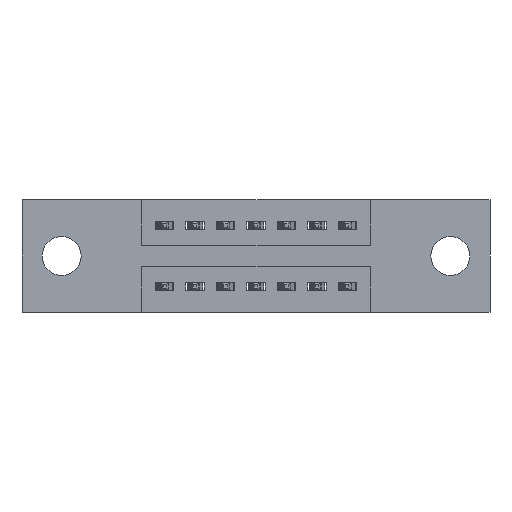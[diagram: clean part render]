
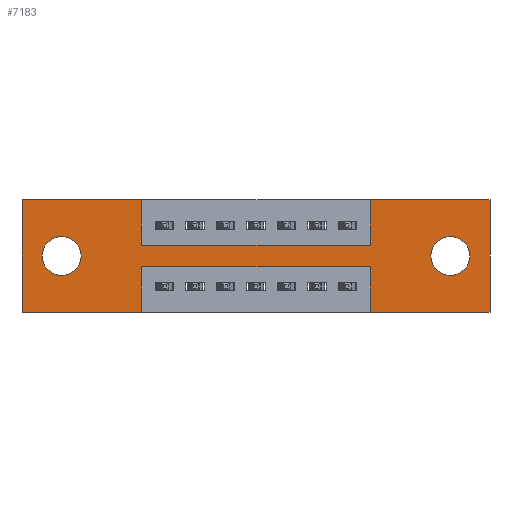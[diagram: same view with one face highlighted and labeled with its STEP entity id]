
A CAD part, front view. The second image highlights one B-rep face of the part: STEP entity #7183.
In plain terms, the highlighted planar face has unit normal (0, -1, 0).
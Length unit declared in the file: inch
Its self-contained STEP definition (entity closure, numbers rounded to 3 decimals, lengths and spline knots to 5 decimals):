
#76 = CARTESIAN_POINT ( 'NONE',  ( 1.535, 0., -0.37 ) ) ;
#187 = CARTESIAN_POINT ( 'NONE',  ( 1.405, 0., -0.121 ) ) ;
#204 = DIRECTION ( 'NONE',  ( 0., 0., 1. ) ) ;
#265 = AXIS2_PLACEMENT_3D ( 'NONE', #5460, #5365, #774 ) ;
#313 = ORIENTED_EDGE ( 'NONE', *, *, #1793, .T. ) ;
#326 = EDGE_CURVE ( 'NONE', #2442, #1435, #8876, .T. ) ;
#570 = EDGE_CURVE ( 'NONE', #6640, #3226, #3095, .T. ) ;
#571 = AXIS2_PLACEMENT_3D ( 'NONE', #7916, #8763, #7945 ) ;
#619 = ORIENTED_EDGE ( 'NONE', *, *, #6736, .F. ) ;
#620 = VECTOR ( 'NONE', #10150, 39.37008 ) ;
#634 = PLANE ( 'NONE',  #265 ) ;
#736 = VERTEX_POINT ( 'NONE', #3620 ) ;
#774 = DIRECTION ( 'NONE',  ( 0., 0., -1. ) ) ;
#858 = EDGE_CURVE ( 'NONE', #7406, #1645, #5656, .T. ) ;
#904 = ORIENTED_EDGE ( 'NONE', *, *, #1548, .F. ) ;
#1179 = EDGE_LOOP ( 'NONE', ( #6719, #5673 ) ) ;
#1204 = LINE ( 'NONE', #7947, #6472 ) ;
#1272 = VECTOR ( 'NONE', #204, 39.37008 ) ;
#1367 = CARTESIAN_POINT ( 'NONE',  ( 1.1425, 0., -0.22 ) ) ;
#1422 = VERTEX_POINT ( 'NONE', #1986 ) ;
#1435 = VERTEX_POINT ( 'NONE', #5290 ) ;
#1548 = EDGE_CURVE ( 'NONE', #7769, #8392, #8644, .T. ) ;
#1588 = VERTEX_POINT ( 'NONE', #10041 ) ;
#1621 = ORIENTED_EDGE ( 'NONE', *, *, #7367, .F. ) ;
#1645 = VERTEX_POINT ( 'NONE', #5626 ) ;
#1672 = EDGE_CURVE ( 'NONE', #1645, #3684, #1204, .T. ) ;
#1702 = DIRECTION ( 'NONE',  ( 0., 0., 1. ) ) ;
#1793 = EDGE_CURVE ( 'NONE', #3226, #6640, #6588, .T. ) ;
#1831 = VERTEX_POINT ( 'NONE', #4804 ) ;
#1974 = AXIS2_PLACEMENT_3D ( 'NONE', #4009, #9537, #6337 ) ;
#1986 = CARTESIAN_POINT ( 'NONE',  ( 1.1425, 0., 0. ) ) ;
#2091 = DIRECTION ( 'NONE',  ( -1., 0., 0. ) ) ;
#2158 = EDGE_CURVE ( 'NONE', #3633, #1831, #3235, .T. ) ;
#2379 = CARTESIAN_POINT ( 'NONE',  ( 0.3925, 0., -0.37 ) ) ;
#2424 = LINE ( 'NONE', #7381, #3416 ) ;
#2442 = VERTEX_POINT ( 'NONE', #76 ) ;
#2478 = DIRECTION ( 'NONE',  ( 0., 0., -1. ) ) ;
#2498 = AXIS2_PLACEMENT_3D ( 'NONE', #7168, #6262, #1702 ) ;
#2695 = LINE ( 'NONE', #8568, #620 ) ;
#2801 = AXIS2_PLACEMENT_3D ( 'NONE', #8997, #4231, #3451 ) ;
#3095 = CIRCLE ( 'NONE', #571, 0.064 ) ;
#3226 = VERTEX_POINT ( 'NONE', #5958 ) ;
#3235 = LINE ( 'NONE', #5209, #8972 ) ;
#3416 = VECTOR ( 'NONE', #6493, 39.37008 ) ;
#3451 = DIRECTION ( 'NONE',  ( 0., 0., 1. ) ) ;
#3563 = ORIENTED_EDGE ( 'NONE', *, *, #326, .F. ) ;
#3620 = CARTESIAN_POINT ( 'NONE',  ( 0.13, 0., -0.249 ) ) ;
#3630 = LINE ( 'NONE', #4315, #6886 ) ;
#3633 = VERTEX_POINT ( 'NONE', #4098 ) ;
#3645 = CARTESIAN_POINT ( 'NONE',  ( 0., 0., -0.37 ) ) ;
#3652 = VECTOR ( 'NONE', #7889, 39.37008 ) ;
#3684 = VERTEX_POINT ( 'NONE', #7980 ) ;
#3808 = ORIENTED_EDGE ( 'NONE', *, *, #9370, .F. ) ;
#3893 = DIRECTION ( 'NONE',  ( -1., 0., 0. ) ) ;
#4009 = CARTESIAN_POINT ( 'NONE',  ( 1.405, 0., -0.185 ) ) ;
#4098 = CARTESIAN_POINT ( 'NONE',  ( 0.3925, 0., -0.15 ) ) ;
#4099 = CARTESIAN_POINT ( 'NONE',  ( 0.13, 0., -0.121 ) ) ;
#4231 = DIRECTION ( 'NONE',  ( 0., 1., 0. ) ) ;
#4315 = CARTESIAN_POINT ( 'NONE',  ( 1.535, 0., 0. ) ) ;
#4366 = CARTESIAN_POINT ( 'NONE',  ( 0., 0., 0. ) ) ;
#4501 = CARTESIAN_POINT ( 'NONE',  ( 0.3925, 0., -0.22 ) ) ;
#4554 = FACE_BOUND ( 'NONE', #6823, .T. ) ;
#4710 = VECTOR ( 'NONE', #8277, 39.37008 ) ;
#4774 = DIRECTION ( 'NONE',  ( 0., 0., 1. ) ) ;
#4804 = CARTESIAN_POINT ( 'NONE',  ( 1.1425, 0., -0.15 ) ) ;
#5135 = VECTOR ( 'NONE', #2478, 39.37008 ) ;
#5209 = CARTESIAN_POINT ( 'NONE',  ( 0.3925, 0., -0.15 ) ) ;
#5290 = CARTESIAN_POINT ( 'NONE',  ( 1.1425, 0., -0.37 ) ) ;
#5318 = CARTESIAN_POINT ( 'NONE',  ( 0.3925, 0., -0.22 ) ) ;
#5365 = DIRECTION ( 'NONE',  ( 0., -1., 0. ) ) ;
#5398 = FACE_BOUND ( 'NONE', #1179, .T. ) ;
#5460 = CARTESIAN_POINT ( 'NONE',  ( 0., 0., -0.37 ) ) ;
#5626 = CARTESIAN_POINT ( 'NONE',  ( 0., 0., -0.37 ) ) ;
#5648 = CARTESIAN_POINT ( 'NONE',  ( 1.1425, 0., -0.37 ) ) ;
#5656 = LINE ( 'NONE', #5968, #7804 ) ;
#5673 = ORIENTED_EDGE ( 'NONE', *, *, #10101, .T. ) ;
#5956 = EDGE_CURVE ( 'NONE', #3684, #1588, #2424, .T. ) ;
#5958 = CARTESIAN_POINT ( 'NONE',  ( 1.405, 0., -0.249 ) ) ;
#5968 = CARTESIAN_POINT ( 'NONE',  ( 0., 0., -0.37 ) ) ;
#5972 = EDGE_CURVE ( 'NONE', #9496, #736, #7125, .T. ) ;
#6105 = ORIENTED_EDGE ( 'NONE', *, *, #570, .T. ) ;
#6245 = CIRCLE ( 'NONE', #2498, 0.064 ) ;
#6262 = DIRECTION ( 'NONE',  ( 0., 1., 0. ) ) ;
#6337 = DIRECTION ( 'NONE',  ( 0., 0., -1. ) ) ;
#6466 = VECTOR ( 'NONE', #10005, 39.37008 ) ;
#6472 = VECTOR ( 'NONE', #4774, 39.37008 ) ;
#6493 = DIRECTION ( 'NONE',  ( 1., 0., 0. ) ) ;
#6557 = LINE ( 'NONE', #5648, #1272 ) ;
#6588 = CIRCLE ( 'NONE', #1974, 0.064 ) ;
#6640 = VERTEX_POINT ( 'NONE', #187 ) ;
#6697 = DIRECTION ( 'NONE',  ( 0., 0., -1. ) ) ;
#6719 = ORIENTED_EDGE ( 'NONE', *, *, #5972, .T. ) ;
#6736 = EDGE_CURVE ( 'NONE', #1435, #7769, #6557, .T. ) ;
#6823 = EDGE_LOOP ( 'NONE', ( #6105, #313 ) ) ;
#6841 = ORIENTED_EDGE ( 'NONE', *, *, #5956, .F. ) ;
#6886 = VECTOR ( 'NONE', #6697, 39.37008 ) ;
#7125 = CIRCLE ( 'NONE', #2801, 0.064 ) ;
#7129 = ORIENTED_EDGE ( 'NONE', *, *, #858, .F. ) ;
#7168 = CARTESIAN_POINT ( 'NONE',  ( 0.13, 0., -0.185 ) ) ;
#7183 = ADVANCED_FACE ( 'NONE', ( #4554, #5398, #8300 ), #634, .T. ) ;
#7187 = ORIENTED_EDGE ( 'NONE', *, *, #1672, .F. ) ;
#7300 = CARTESIAN_POINT ( 'NONE',  ( 0.3925, 0., -0.37 ) ) ;
#7367 = EDGE_CURVE ( 'NONE', #1588, #3633, #8810, .T. ) ;
#7381 = CARTESIAN_POINT ( 'NONE',  ( 0., 0., 0. ) ) ;
#7406 = VERTEX_POINT ( 'NONE', #7300 ) ;
#7512 = EDGE_CURVE ( 'NONE', #1422, #9919, #10200, .T. ) ;
#7709 = EDGE_LOOP ( 'NONE', ( #8619, #904, #619, #3563, #3808, #7728, #8996, #8426, #1621, #6841, #7187, #7129 ) ) ;
#7728 = ORIENTED_EDGE ( 'NONE', *, *, #7512, .F. ) ;
#7769 = VERTEX_POINT ( 'NONE', #1367 ) ;
#7804 = VECTOR ( 'NONE', #2091, 39.37008 ) ;
#7873 = VECTOR ( 'NONE', #3893, 39.37008 ) ;
#7889 = DIRECTION ( 'NONE',  ( 0., 0., -1. ) ) ;
#7916 = CARTESIAN_POINT ( 'NONE',  ( 1.405, 0., -0.185 ) ) ;
#7945 = DIRECTION ( 'NONE',  ( 0., 0., -1. ) ) ;
#7947 = CARTESIAN_POINT ( 'NONE',  ( 0., 0., 0. ) ) ;
#7980 = CARTESIAN_POINT ( 'NONE',  ( 0., 0., 0. ) ) ;
#8232 = DIRECTION ( 'NONE',  ( 1., 0., 0. ) ) ;
#8277 = DIRECTION ( 'NONE',  ( 1., 0., 0. ) ) ;
#8300 = FACE_OUTER_BOUND ( 'NONE', #7709, .T. ) ;
#8392 = VERTEX_POINT ( 'NONE', #5318 ) ;
#8426 = ORIENTED_EDGE ( 'NONE', *, *, #2158, .F. ) ;
#8568 = CARTESIAN_POINT ( 'NONE',  ( 1.1425, 0., 0. ) ) ;
#8619 = ORIENTED_EDGE ( 'NONE', *, *, #9625, .F. ) ;
#8644 = LINE ( 'NONE', #4501, #7873 ) ;
#8763 = DIRECTION ( 'NONE',  ( 0., 1., 0. ) ) ;
#8769 = CARTESIAN_POINT ( 'NONE',  ( 0.3925, 0., 0. ) ) ;
#8810 = LINE ( 'NONE', #8769, #5135 ) ;
#8876 = LINE ( 'NONE', #3645, #6466 ) ;
#8893 = CARTESIAN_POINT ( 'NONE',  ( 1.535, 0., 0. ) ) ;
#8972 = VECTOR ( 'NONE', #8232, 39.37008 ) ;
#8996 = ORIENTED_EDGE ( 'NONE', *, *, #9961, .F. ) ;
#8997 = CARTESIAN_POINT ( 'NONE',  ( 0.13, 0., -0.185 ) ) ;
#9370 = EDGE_CURVE ( 'NONE', #9919, #2442, #3630, .T. ) ;
#9496 = VERTEX_POINT ( 'NONE', #4099 ) ;
#9537 = DIRECTION ( 'NONE',  ( 0., 1., 0. ) ) ;
#9625 = EDGE_CURVE ( 'NONE', #8392, #7406, #9958, .T. ) ;
#9919 = VERTEX_POINT ( 'NONE', #8893 ) ;
#9958 = LINE ( 'NONE', #2379, #3652 ) ;
#9961 = EDGE_CURVE ( 'NONE', #1831, #1422, #2695, .T. ) ;
#10005 = DIRECTION ( 'NONE',  ( -1., 0., 0. ) ) ;
#10041 = CARTESIAN_POINT ( 'NONE',  ( 0.3925, 0., 0. ) ) ;
#10101 = EDGE_CURVE ( 'NONE', #736, #9496, #6245, .T. ) ;
#10150 = DIRECTION ( 'NONE',  ( 0., 0., 1. ) ) ;
#10200 = LINE ( 'NONE', #4366, #4710 ) ;
